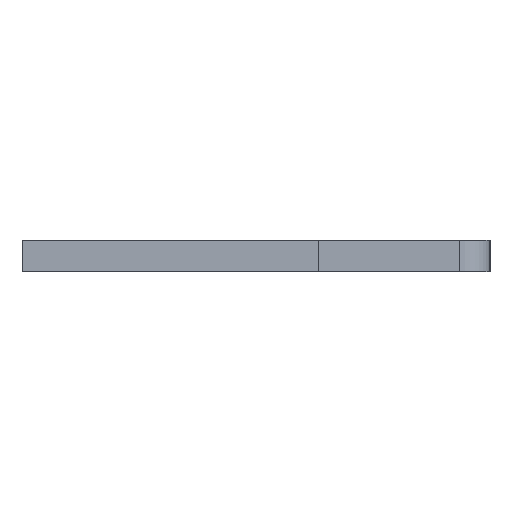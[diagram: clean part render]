
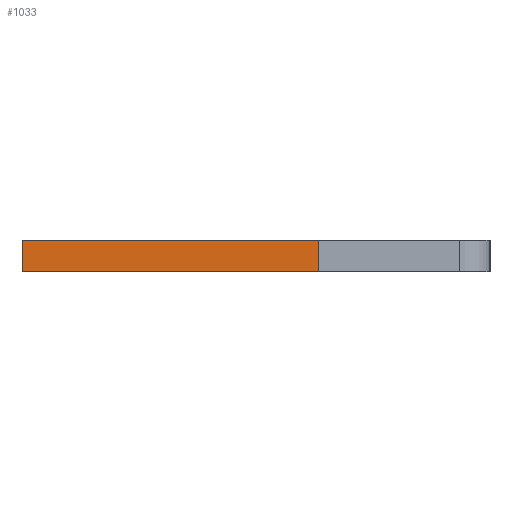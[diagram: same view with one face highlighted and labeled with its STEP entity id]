
A CAD part, left-side view. The second image highlights one B-rep face of the part: STEP entity #1033.
In plain terms, the highlighted face is planar.
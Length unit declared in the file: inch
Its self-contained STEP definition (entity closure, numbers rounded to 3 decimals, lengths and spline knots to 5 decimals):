
#28 = LINE ( 'NONE', #505, #388 ) ;
#42 = VERTEX_POINT ( 'NONE', #798 ) ;
#58 = DIRECTION ( 'NONE',  ( 0., 1., 0. ) ) ;
#62 = CARTESIAN_POINT ( 'NONE',  ( -0.01, 0.15, -0.04 ) ) ;
#92 = DIRECTION ( 'NONE',  ( -1., 0., 0. ) ) ;
#95 = VERTEX_POINT ( 'NONE', #62 ) ;
#152 = DIRECTION ( 'NONE',  ( 0., 1., 0. ) ) ;
#252 = CARTESIAN_POINT ( 'NONE',  ( 0.01, 0.15, -0.04 ) ) ;
#261 = CARTESIAN_POINT ( 'NONE',  ( 0.01, 0.15, -0.04 ) ) ;
#262 = CARTESIAN_POINT ( 'NONE',  ( 0.01, -0.04, -0.04 ) ) ;
#276 = EDGE_CURVE ( 'NONE', #740, #95, #637, .T. ) ;
#361 = EDGE_CURVE ( 'NONE', #42, #95, #807, .T. ) ;
#381 = ORIENTED_EDGE ( 'NONE', *, *, #442, .F. ) ;
#388 = VECTOR ( 'NONE', #152, 39.37008 ) ;
#401 = VECTOR ( 'NONE', #58, 39.37008 ) ;
#442 = EDGE_CURVE ( 'NONE', #1071, #42, #28, .T. ) ;
#445 = CARTESIAN_POINT ( 'NONE',  ( 0.01, -0.04, -0.04 ) ) ;
#453 = LINE ( 'NONE', #445, #741 ) ;
#460 = EDGE_LOOP ( 'NONE', ( #1003, #1019, #381, #585 ) ) ;
#505 = CARTESIAN_POINT ( 'NONE',  ( 0.01, 0.15, -0.04 ) ) ;
#585 = ORIENTED_EDGE ( 'NONE', *, *, #683, .T. ) ;
#598 = PLANE ( 'NONE',  #704 ) ;
#637 = LINE ( 'NONE', #991, #401 ) ;
#658 = VECTOR ( 'NONE', #761, 39.37008 ) ;
#683 = EDGE_CURVE ( 'NONE', #1071, #740, #453, .T. ) ;
#704 = AXIS2_PLACEMENT_3D ( 'NONE', #252, #838, #928 ) ;
#740 = VERTEX_POINT ( 'NONE', #967 ) ;
#741 = VECTOR ( 'NONE', #92, 39.37008 ) ;
#761 = DIRECTION ( 'NONE',  ( -1., 0., 0. ) ) ;
#798 = CARTESIAN_POINT ( 'NONE',  ( 0.01, 0.15, -0.04 ) ) ;
#807 = LINE ( 'NONE', #261, #658 ) ;
#838 = DIRECTION ( 'NONE',  ( 0., 0., 1. ) ) ;
#928 = DIRECTION ( 'NONE',  ( 1., 0., 0. ) ) ;
#967 = CARTESIAN_POINT ( 'NONE',  ( -0.01, -0.04, -0.04 ) ) ;
#991 = CARTESIAN_POINT ( 'NONE',  ( -0.01, 0.15, -0.04 ) ) ;
#1003 = ORIENTED_EDGE ( 'NONE', *, *, #276, .T. ) ;
#1019 = ORIENTED_EDGE ( 'NONE', *, *, #361, .F. ) ;
#1033 = ADVANCED_FACE ( 'NONE', ( #1045 ), #598, .F. ) ;
#1045 = FACE_OUTER_BOUND ( 'NONE', #460, .T. ) ;
#1071 = VERTEX_POINT ( 'NONE', #262 ) ;
